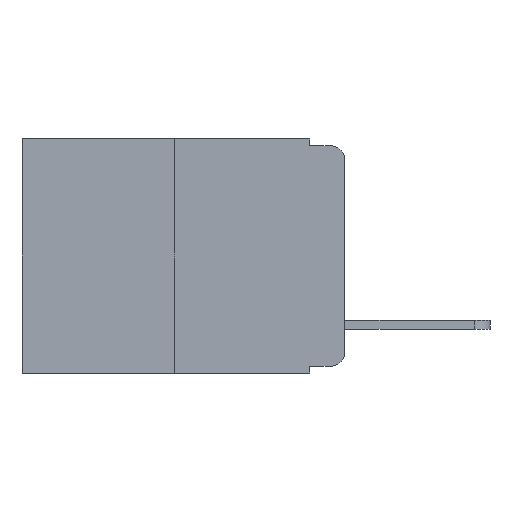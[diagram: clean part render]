
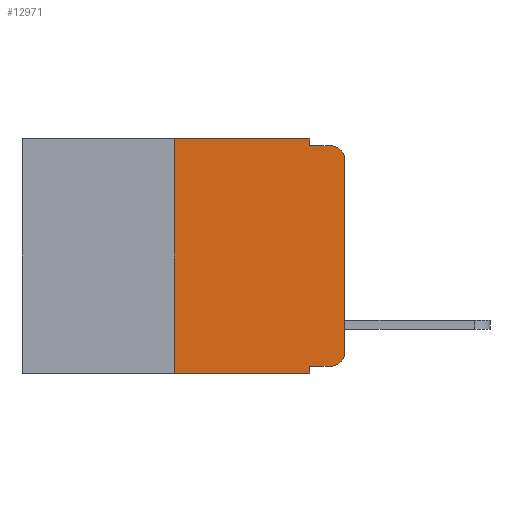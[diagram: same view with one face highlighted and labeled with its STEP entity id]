
A CAD part, left-side view. The second image highlights one B-rep face of the part: STEP entity #12971.
In plain terms, the highlighted planar face has unit normal (-1, 0, 0).
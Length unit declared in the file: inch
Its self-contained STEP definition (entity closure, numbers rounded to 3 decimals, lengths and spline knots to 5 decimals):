
#42 = AXIS2_PLACEMENT_3D ( 'NONE', #1069, #23740, #13046 ) ;
#61 = VERTEX_POINT ( 'NONE', #8421 ) ;
#493 = VERTEX_POINT ( 'NONE', #2829 ) ;
#593 = DIRECTION ( 'NONE',  ( 0., -1., 0. ) ) ;
#1069 = CARTESIAN_POINT ( 'NONE',  ( 0., 0.02, -0.03 ) ) ;
#2039 = LINE ( 'NONE', #6183, #25053 ) ;
#2247 = DIRECTION ( 'NONE',  ( 0., 0., -1. ) ) ;
#2580 = EDGE_CURVE ( 'NONE', #15927, #493, #26095, .T. ) ;
#2751 = LINE ( 'NONE', #22578, #7993 ) ;
#2829 = CARTESIAN_POINT ( 'NONE',  ( 0., 0.051, 0. ) ) ;
#3534 = CARTESIAN_POINT ( 'NONE',  ( 0., 0.25, -0.343 ) ) ;
#4910 = VECTOR ( 'NONE', #2247, 39.37008 ) ;
#5006 = PLANE ( 'NONE',  #18031 ) ;
#5619 = ORIENTED_EDGE ( 'NONE', *, *, #6792, .T. ) ;
#6183 = CARTESIAN_POINT ( 'NONE',  ( 0., 0.051, -0.01 ) ) ;
#6292 = VECTOR ( 'NONE', #593, 39.37008 ) ;
#6375 = ORIENTED_EDGE ( 'NONE', *, *, #11382, .T. ) ;
#6496 = VERTEX_POINT ( 'NONE', #19720 ) ;
#6792 = EDGE_CURVE ( 'NONE', #20493, #10797, #11436, .T. ) ;
#7477 = VECTOR ( 'NONE', #17977, 39.37008 ) ;
#7745 = VERTEX_POINT ( 'NONE', #24880 ) ;
#7993 = VECTOR ( 'NONE', #22665, 39.37008 ) ;
#8421 = CARTESIAN_POINT ( 'NONE',  ( 0., 0.051, -0.01 ) ) ;
#8926 = DIRECTION ( 'NONE',  ( 0., 0., -1. ) ) ;
#9031 = CARTESIAN_POINT ( 'NONE',  ( 0., 0.473, 0. ) ) ;
#9542 = CARTESIAN_POINT ( 'NONE',  ( 0., 0.02, -0.333 ) ) ;
#9817 = LINE ( 'NONE', #23294, #4910 ) ;
#10560 = ORIENTED_EDGE ( 'NONE', *, *, #10611, .T. ) ;
#10611 = EDGE_CURVE ( 'NONE', #19012, #22892, #25858, .T. ) ;
#10709 = LINE ( 'NONE', #11991, #15887 ) ;
#10797 = VERTEX_POINT ( 'NONE', #19733 ) ;
#11382 = EDGE_CURVE ( 'NONE', #10797, #19012, #25141, .T. ) ;
#11436 = CIRCLE ( 'NONE', #23986, 0.02 ) ;
#11442 = VERTEX_POINT ( 'NONE', #3534 ) ;
#11517 = ORIENTED_EDGE ( 'NONE', *, *, #16498, .T. ) ;
#11612 = ORIENTED_EDGE ( 'NONE', *, *, #25309, .F. ) ;
#11881 = CARTESIAN_POINT ( 'NONE',  ( 0., 0.25, 0. ) ) ;
#11991 = CARTESIAN_POINT ( 'NONE',  ( 0., 0.051, 0. ) ) ;
#12333 = DIRECTION ( 'NONE',  ( 0., 0., -1. ) ) ;
#12613 = EDGE_CURVE ( 'NONE', #493, #61, #9817, .T. ) ;
#12971 = ADVANCED_FACE ( 'NONE', ( #21474 ), #5006, .F. ) ;
#13046 = DIRECTION ( 'NONE',  ( 0., 0., -1. ) ) ;
#13476 = DIRECTION ( 'NONE',  ( 0., 0., -1. ) ) ;
#14528 = EDGE_LOOP ( 'NONE', ( #6375, #10560, #15651, #24986, #24304, #11612, #11517, #14773, #25395, #5619 ) ) ;
#14773 = ORIENTED_EDGE ( 'NONE', *, *, #21657, .F. ) ;
#15651 = ORIENTED_EDGE ( 'NONE', *, *, #20027, .F. ) ;
#15887 = VECTOR ( 'NONE', #12333, 39.37008 ) ;
#15927 = VERTEX_POINT ( 'NONE', #18161 ) ;
#15943 = DIRECTION ( 'NONE',  ( 0., 0., 1. ) ) ;
#16498 = EDGE_CURVE ( 'NONE', #11442, #6496, #22949, .T. ) ;
#17418 = VECTOR ( 'NONE', #20288, 39.37008 ) ;
#17487 = CARTESIAN_POINT ( 'NONE',  ( 0., 0.02, -0.313 ) ) ;
#17977 = DIRECTION ( 'NONE',  ( 0., 0., 1. ) ) ;
#18031 = AXIS2_PLACEMENT_3D ( 'NONE', #25688, #25410, #8926 ) ;
#18060 = VECTOR ( 'NONE', #15943, 39.37008 ) ;
#18161 = CARTESIAN_POINT ( 'NONE',  ( 0., 0.25, 0. ) ) ;
#19012 = VERTEX_POINT ( 'NONE', #19211 ) ;
#19211 = CARTESIAN_POINT ( 'NONE',  ( 0., 0., -0.03 ) ) ;
#19456 = CARTESIAN_POINT ( 'NONE',  ( 0., 0.02, -0.01 ) ) ;
#19720 = CARTESIAN_POINT ( 'NONE',  ( 0., 0.051, -0.343 ) ) ;
#19733 = CARTESIAN_POINT ( 'NONE',  ( 0., 0., -0.313 ) ) ;
#20012 = CARTESIAN_POINT ( 'NONE',  ( 0., 0.473, -0.343 ) ) ;
#20027 = EDGE_CURVE ( 'NONE', #61, #22892, #2039, .T. ) ;
#20288 = DIRECTION ( 'NONE',  ( 0., -1., 0. ) ) ;
#20493 = VERTEX_POINT ( 'NONE', #9542 ) ;
#20715 = DIRECTION ( 'NONE',  ( 0., -1., 0. ) ) ;
#21474 = FACE_OUTER_BOUND ( 'NONE', #14528, .T. ) ;
#21657 = EDGE_CURVE ( 'NONE', #7745, #6496, #10709, .T. ) ;
#22578 = CARTESIAN_POINT ( 'NONE',  ( 0., 0.051, -0.333 ) ) ;
#22665 = DIRECTION ( 'NONE',  ( 0., -1., 0. ) ) ;
#22892 = VERTEX_POINT ( 'NONE', #19456 ) ;
#22949 = LINE ( 'NONE', #20012, #17418 ) ;
#23294 = CARTESIAN_POINT ( 'NONE',  ( 0., 0.051, 0. ) ) ;
#23740 = DIRECTION ( 'NONE',  ( -1., 0., 0. ) ) ;
#23966 = EDGE_CURVE ( 'NONE', #7745, #20493, #2751, .T. ) ;
#23986 = AXIS2_PLACEMENT_3D ( 'NONE', #17487, #25908, #13476 ) ;
#24304 = ORIENTED_EDGE ( 'NONE', *, *, #2580, .F. ) ;
#24669 = LINE ( 'NONE', #11881, #7477 ) ;
#24880 = CARTESIAN_POINT ( 'NONE',  ( 0., 0.051, -0.333 ) ) ;
#24986 = ORIENTED_EDGE ( 'NONE', *, *, #12613, .F. ) ;
#25053 = VECTOR ( 'NONE', #20715, 39.37008 ) ;
#25141 = LINE ( 'NONE', #26293, #18060 ) ;
#25309 = EDGE_CURVE ( 'NONE', #11442, #15927, #24669, .T. ) ;
#25395 = ORIENTED_EDGE ( 'NONE', *, *, #23966, .T. ) ;
#25410 = DIRECTION ( 'NONE',  ( 1., 0., 0. ) ) ;
#25688 = CARTESIAN_POINT ( 'NONE',  ( 0., 0.473, 0. ) ) ;
#25858 = CIRCLE ( 'NONE', #42, 0.02 ) ;
#25908 = DIRECTION ( 'NONE',  ( -1., 0., 0. ) ) ;
#26095 = LINE ( 'NONE', #9031, #6292 ) ;
#26293 = CARTESIAN_POINT ( 'NONE',  ( 0., 0., 0. ) ) ;
